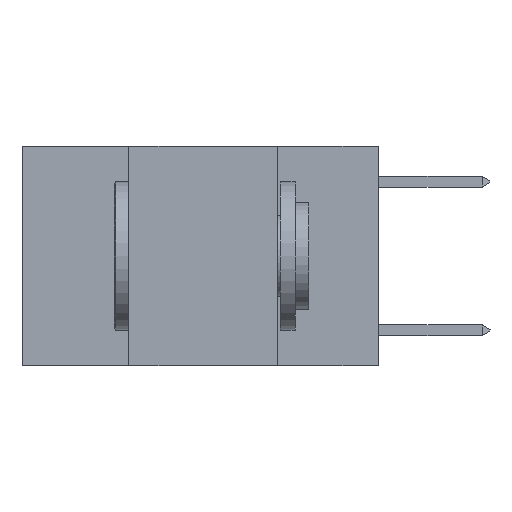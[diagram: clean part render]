
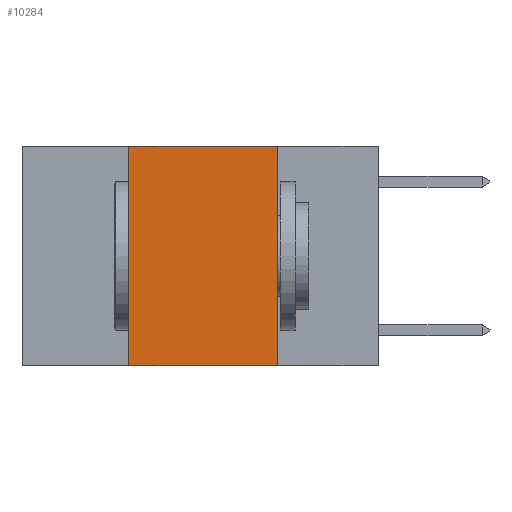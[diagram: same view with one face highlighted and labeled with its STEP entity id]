
A CAD part, left-side view. The second image highlights one B-rep face of the part: STEP entity #10284.
In plain terms, the highlighted planar face has unit normal (-1, 0, 0).
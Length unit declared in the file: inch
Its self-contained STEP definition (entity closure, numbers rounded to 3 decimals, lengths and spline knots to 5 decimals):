
#1204 = LINE ( 'NONE', #8624, #5971 ) ;
#1892 = LINE ( 'NONE', #25703, #12004 ) ;
#4457 = VECTOR ( 'NONE', #8598, 39.37008 ) ;
#5532 = LINE ( 'NONE', #9586, #15637 ) ;
#5892 = EDGE_CURVE ( 'NONE', #18795, #19823, #5532, .T. ) ;
#5971 = VECTOR ( 'NONE', #18733, 39.37008 ) ;
#7610 = DIRECTION ( 'NONE',  ( 0., 0., -1. ) ) ;
#7644 = DIRECTION ( 'NONE',  ( 1., 0., 0. ) ) ;
#7647 = CARTESIAN_POINT ( 'NONE',  ( 0., 0.6, 0. ) ) ;
#7828 = CARTESIAN_POINT ( 'NONE',  ( 0., 0.17, 0. ) ) ;
#8174 = FACE_OUTER_BOUND ( 'NONE', #13759, .T. ) ;
#8208 = PLANE ( 'NONE',  #16583 ) ;
#8213 = CARTESIAN_POINT ( 'NONE',  ( 0., 0.42, -0.37 ) ) ;
#8598 = DIRECTION ( 'NONE',  ( 0., 0., -1. ) ) ;
#8624 = CARTESIAN_POINT ( 'NONE',  ( 0., 0.42, 0. ) ) ;
#9067 = ORIENTED_EDGE ( 'NONE', *, *, #11918, .F. ) ;
#9238 = EDGE_CURVE ( 'NONE', #10267, #17540, #1892, .T. ) ;
#9586 = CARTESIAN_POINT ( 'NONE',  ( 0., 0.6, 0. ) ) ;
#10267 = VERTEX_POINT ( 'NONE', #8213 ) ;
#10284 = ADVANCED_FACE ( 'NONE', ( #8174 ), #8208, .F. ) ;
#11918 = EDGE_CURVE ( 'NONE', #10267, #18795, #1204, .T. ) ;
#12004 = VECTOR ( 'NONE', #25643, 39.37008 ) ;
#13759 = EDGE_LOOP ( 'NONE', ( #14746, #24160, #9067, #19974 ) ) ;
#14746 = ORIENTED_EDGE ( 'NONE', *, *, #25580, .F. ) ;
#15263 = CARTESIAN_POINT ( 'NONE',  ( 0., 0.17, -0.37 ) ) ;
#15637 = VECTOR ( 'NONE', #25946, 39.37008 ) ;
#16583 = AXIS2_PLACEMENT_3D ( 'NONE', #7647, #7644, #7610 ) ;
#16999 = CARTESIAN_POINT ( 'NONE',  ( 0., 0.42, 0. ) ) ;
#17540 = VERTEX_POINT ( 'NONE', #15263 ) ;
#18712 = CARTESIAN_POINT ( 'NONE',  ( 0., 0.17, 0. ) ) ;
#18733 = DIRECTION ( 'NONE',  ( 0., 0., 1. ) ) ;
#18795 = VERTEX_POINT ( 'NONE', #16999 ) ;
#19823 = VERTEX_POINT ( 'NONE', #7828 ) ;
#19974 = ORIENTED_EDGE ( 'NONE', *, *, #9238, .T. ) ;
#24160 = ORIENTED_EDGE ( 'NONE', *, *, #5892, .F. ) ;
#25408 = LINE ( 'NONE', #18712, #4457 ) ;
#25580 = EDGE_CURVE ( 'NONE', #19823, #17540, #25408, .T. ) ;
#25643 = DIRECTION ( 'NONE',  ( 0., -1., 0. ) ) ;
#25703 = CARTESIAN_POINT ( 'NONE',  ( 0., 0.6, -0.37 ) ) ;
#25946 = DIRECTION ( 'NONE',  ( 0., -1., 0. ) ) ;
